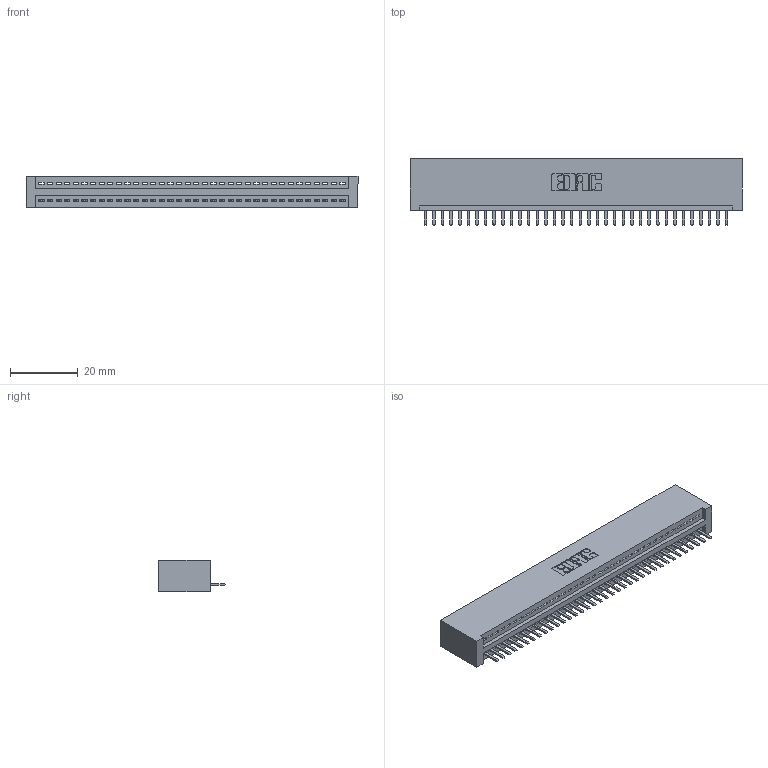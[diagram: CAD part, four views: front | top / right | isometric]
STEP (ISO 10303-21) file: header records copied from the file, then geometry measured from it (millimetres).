
FILE_DESCRIPTION (( 'STEP AP203' ), '1' );
FILE_NAME ('345-036-520-101.STEP', '2019-10-07T22:13:16', ( '' ), ( '' ), 'SwSTEP 2.0', 'SolidWorks 2016', '' );
FILE_SCHEMA (( 'CONFIG_CONTROL_DESIGN' ));
Length unit declared in the file: inch
Products named in the file (3): 345-292-001_345-293-120; 345-036-520-101; 345 Part_No Mounting Lugs
Assembly tree (37 placements, depth 2):
  345-036-520-101
    345 Part_No Mounting Lugs
    345-292-001_345-293-120  x36
Bounding box: 98.04 x 19.68 x 9.4 mm (x, y, z)
Volume: 9744 mm3; surface area: 12718.7 mm2
Topology: 37 solids, 37 shells, 2350 faces, 6941 edges, 4530 vertices
Faces by surface type: plane 1588, cylinder 762
Entity records: 27739 total; most frequent: CARTESIAN_POINT 4824, ORIENTED_EDGE 4782, DIRECTION 4203, EDGE_CURVE 2391, LINE 2119, VECTOR 2119, VERTEX_POINT 1590, AXIS2_PLACEMENT_3D 1042
